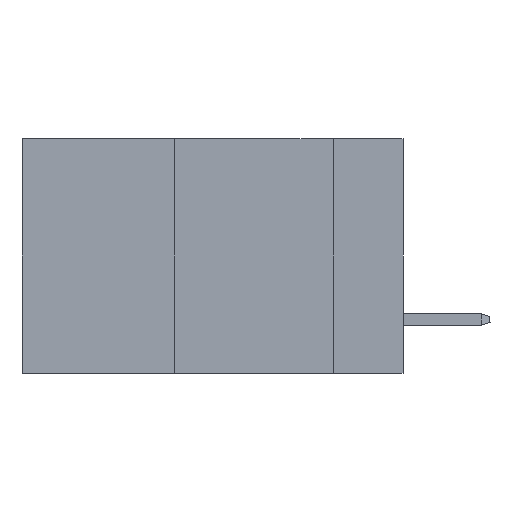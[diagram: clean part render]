
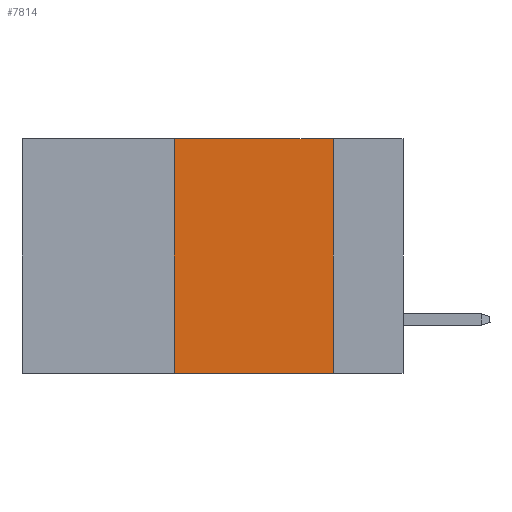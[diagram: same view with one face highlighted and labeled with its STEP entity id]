
A CAD part, left-side view. The second image highlights one B-rep face of the part: STEP entity #7814.
In plain terms, the highlighted planar face has unit normal (-1, 0, 0).
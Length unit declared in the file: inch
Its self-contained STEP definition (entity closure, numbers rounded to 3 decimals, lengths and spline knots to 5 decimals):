
#1609 = VECTOR ( 'NONE', #5691, 39.37008 ) ;
#2542 = ORIENTED_EDGE ( 'NONE', *, *, #4721, .F. ) ;
#2997 = VECTOR ( 'NONE', #13580, 39.37008 ) ;
#3041 = ORIENTED_EDGE ( 'NONE', *, *, #21338, .F. ) ;
#3116 = LINE ( 'NONE', #14403, #17725 ) ;
#4425 = DIRECTION ( 'NONE',  ( 0., 0., -1. ) ) ;
#4721 = EDGE_CURVE ( 'NONE', #5520, #15508, #15247, .T. ) ;
#5422 = CARTESIAN_POINT ( 'NONE',  ( 0., 0.36, -0.37 ) ) ;
#5520 = VERTEX_POINT ( 'NONE', #5422 ) ;
#5691 = DIRECTION ( 'NONE',  ( 0., -1., 0. ) ) ;
#7699 = CARTESIAN_POINT ( 'NONE',  ( 0., 0.11, -0.37 ) ) ;
#7814 = ADVANCED_FACE ( 'NONE', ( #9763 ), #20562, .F. ) ;
#7993 = VECTOR ( 'NONE', #21757, 39.37008 ) ;
#8233 = ORIENTED_EDGE ( 'NONE', *, *, #13227, .F. ) ;
#9333 = CARTESIAN_POINT ( 'NONE',  ( 0., 0.6, -0.37 ) ) ;
#9451 = AXIS2_PLACEMENT_3D ( 'NONE', #20901, #22594, #4425 ) ;
#9763 = FACE_OUTER_BOUND ( 'NONE', #21476, .T. ) ;
#13227 = EDGE_CURVE ( 'NONE', #15508, #21839, #3116, .T. ) ;
#13580 = DIRECTION ( 'NONE',  ( 0., 0., 1. ) ) ;
#14403 = CARTESIAN_POINT ( 'NONE',  ( 0., 0.6, 0. ) ) ;
#14629 = LINE ( 'NONE', #21993, #7993 ) ;
#14680 = EDGE_CURVE ( 'NONE', #5520, #19002, #22163, .T. ) ;
#15247 = LINE ( 'NONE', #15376, #2997 ) ;
#15376 = CARTESIAN_POINT ( 'NONE',  ( 0., 0.36, 0. ) ) ;
#15508 = VERTEX_POINT ( 'NONE', #22074 ) ;
#15741 = ORIENTED_EDGE ( 'NONE', *, *, #14680, .T. ) ;
#16096 = DIRECTION ( 'NONE',  ( 0., -1., 0. ) ) ;
#17725 = VECTOR ( 'NONE', #16096, 39.37008 ) ;
#18857 = CARTESIAN_POINT ( 'NONE',  ( 0., 0.11, 0. ) ) ;
#19002 = VERTEX_POINT ( 'NONE', #7699 ) ;
#20562 = PLANE ( 'NONE',  #9451 ) ;
#20901 = CARTESIAN_POINT ( 'NONE',  ( 0., 0.6, 0. ) ) ;
#21338 = EDGE_CURVE ( 'NONE', #21839, #19002, #14629, .T. ) ;
#21476 = EDGE_LOOP ( 'NONE', ( #3041, #8233, #2542, #15741 ) ) ;
#21757 = DIRECTION ( 'NONE',  ( 0., 0., -1. ) ) ;
#21839 = VERTEX_POINT ( 'NONE', #18857 ) ;
#21993 = CARTESIAN_POINT ( 'NONE',  ( 0., 0.11, 0. ) ) ;
#22074 = CARTESIAN_POINT ( 'NONE',  ( 0., 0.36, 0. ) ) ;
#22163 = LINE ( 'NONE', #9333, #1609 ) ;
#22594 = DIRECTION ( 'NONE',  ( 1., 0., 0. ) ) ;
